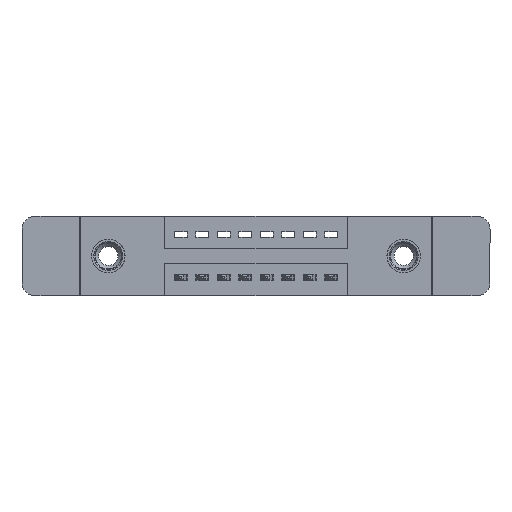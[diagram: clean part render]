
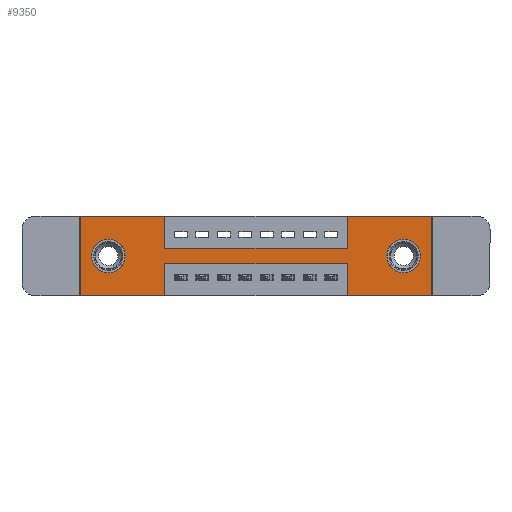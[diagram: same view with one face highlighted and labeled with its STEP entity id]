
A CAD part, front view. The second image highlights one B-rep face of the part: STEP entity #9350.
In plain terms, the highlighted planar face has unit normal (0, -1, 0).
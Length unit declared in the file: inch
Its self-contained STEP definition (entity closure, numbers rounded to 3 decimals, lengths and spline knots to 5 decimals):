
#38 = CARTESIAN_POINT ( 'NONE',  ( 0., 0., 0. ) ) ;
#40 = EDGE_CURVE ( 'NONE', #2316, #5330, #7131, .T. ) ;
#56 = ORIENTED_EDGE ( 'NONE', *, *, #5959, .T. ) ;
#145 = VERTEX_POINT ( 'NONE', #13485 ) ;
#184 = CARTESIAN_POINT ( 'NONE',  ( 0., 0., -0.37 ) ) ;
#198 = EDGE_CURVE ( 'NONE', #11744, #13401, #5810, .T. ) ;
#354 = DIRECTION ( 'NONE',  ( -1., 0., 0. ) ) ;
#569 = CARTESIAN_POINT ( 'NONE',  ( 0.3925, 0., -0.37 ) ) ;
#600 = LINE ( 'NONE', #2339, #7487 ) ;
#678 = VERTEX_POINT ( 'NONE', #4739 ) ;
#805 = EDGE_LOOP ( 'NONE', ( #56, #7225 ) ) ;
#812 = CARTESIAN_POINT ( 'NONE',  ( 0., 0., -0.37 ) ) ;
#832 = LINE ( 'NONE', #38, #14761 ) ;
#871 = AXIS2_PLACEMENT_3D ( 'NONE', #6582, #8857, #4080 ) ;
#1238 = CARTESIAN_POINT ( 'NONE',  ( 1.2425, 0., -0.37 ) ) ;
#1443 = VERTEX_POINT ( 'NONE', #184 ) ;
#1510 = LINE ( 'NONE', #14912, #8026 ) ;
#1944 = CARTESIAN_POINT ( 'NONE',  ( 0.3925, 0., 0. ) ) ;
#2105 = VECTOR ( 'NONE', #10865, 39.37008 ) ;
#2150 = ORIENTED_EDGE ( 'NONE', *, *, #6240, .F. ) ;
#2282 = LINE ( 'NONE', #8129, #6300 ) ;
#2306 = DIRECTION ( 'NONE',  ( 0., 1., 0. ) ) ;
#2316 = VERTEX_POINT ( 'NONE', #6868 ) ;
#2339 = CARTESIAN_POINT ( 'NONE',  ( 0., 0., 0. ) ) ;
#2382 = VECTOR ( 'NONE', #11818, 39.37008 ) ;
#2751 = PLANE ( 'NONE',  #11039 ) ;
#2849 = AXIS2_PLACEMENT_3D ( 'NONE', #15783, #6007, #8430 ) ;
#2877 = EDGE_CURVE ( 'NONE', #6434, #7371, #2282, .T. ) ;
#2977 = VECTOR ( 'NONE', #11588, 39.37008 ) ;
#3133 = VERTEX_POINT ( 'NONE', #12393 ) ;
#3241 = CARTESIAN_POINT ( 'NONE',  ( 0.3925, 0., -0.37 ) ) ;
#3244 = VERTEX_POINT ( 'NONE', #3241 ) ;
#3394 = DIRECTION ( 'NONE',  ( 0., 1., 0. ) ) ;
#3525 = ORIENTED_EDGE ( 'NONE', *, *, #13629, .F. ) ;
#3572 = ORIENTED_EDGE ( 'NONE', *, *, #12669, .T. ) ;
#3719 = VECTOR ( 'NONE', #15218, 39.37008 ) ;
#3744 = ORIENTED_EDGE ( 'NONE', *, *, #6843, .F. ) ;
#4080 = DIRECTION ( 'NONE',  ( 0., 0., -1. ) ) ;
#4309 = ORIENTED_EDGE ( 'NONE', *, *, #15474, .F. ) ;
#4440 = CARTESIAN_POINT ( 'NONE',  ( 0.3925, 0., -0.15 ) ) ;
#4549 = CARTESIAN_POINT ( 'NONE',  ( 0.3925, 0., -0.22 ) ) ;
#4686 = CARTESIAN_POINT ( 'NONE',  ( 0.13, 0., -0.107 ) ) ;
#4704 = DIRECTION ( 'NONE',  ( 0., 0., 1. ) ) ;
#4723 = CIRCLE ( 'NONE', #871, 0.078 ) ;
#4738 = CARTESIAN_POINT ( 'NONE',  ( 0.13, 0., -0.185 ) ) ;
#4739 = CARTESIAN_POINT ( 'NONE',  ( 0., 0., 0. ) ) ;
#5189 = EDGE_LOOP ( 'NONE', ( #3572, #11184 ) ) ;
#5231 = EDGE_LOOP ( 'NONE', ( #10659, #2150, #4309, #3525, #3744, #13785, #8431, #14929, #11423, #13357, #9660, #7241 ) ) ;
#5330 = VERTEX_POINT ( 'NONE', #15211 ) ;
#5810 = CIRCLE ( 'NONE', #9641, 0.078 ) ;
#5941 = LINE ( 'NONE', #569, #10884 ) ;
#5959 = EDGE_CURVE ( 'NONE', #145, #12391, #15179, .T. ) ;
#6007 = DIRECTION ( 'NONE',  ( 0., 1., 0. ) ) ;
#6098 = EDGE_CURVE ( 'NONE', #12391, #145, #4723, .T. ) ;
#6240 = EDGE_CURVE ( 'NONE', #12319, #15354, #14007, .T. ) ;
#6300 = VECTOR ( 'NONE', #13963, 39.37008 ) ;
#6356 = DIRECTION ( 'NONE',  ( 1., 0., 0. ) ) ;
#6434 = VERTEX_POINT ( 'NONE', #10981 ) ;
#6478 = DIRECTION ( 'NONE',  ( 0., -1., 0. ) ) ;
#6488 = VERTEX_POINT ( 'NONE', #15559 ) ;
#6582 = CARTESIAN_POINT ( 'NONE',  ( 1.505, 0., -0.185 ) ) ;
#6825 = FACE_OUTER_BOUND ( 'NONE', #5231, .T. ) ;
#6843 = EDGE_CURVE ( 'NONE', #13503, #3133, #7913, .T. ) ;
#6868 = CARTESIAN_POINT ( 'NONE',  ( 0.3925, 0., 0. ) ) ;
#6890 = DIRECTION ( 'NONE',  ( -1., 0., 0. ) ) ;
#7074 = EDGE_CURVE ( 'NONE', #1443, #678, #14574, .T. ) ;
#7131 = LINE ( 'NONE', #1944, #13185 ) ;
#7144 = CARTESIAN_POINT ( 'NONE',  ( 1.2425, 0., -0.22 ) ) ;
#7225 = ORIENTED_EDGE ( 'NONE', *, *, #6098, .T. ) ;
#7241 = ORIENTED_EDGE ( 'NONE', *, *, #10597, .F. ) ;
#7371 = VERTEX_POINT ( 'NONE', #10656 ) ;
#7487 = VECTOR ( 'NONE', #12174, 39.37008 ) ;
#7728 = VECTOR ( 'NONE', #13560, 39.37008 ) ;
#7837 = DIRECTION ( 'NONE',  ( 0., 0., -1. ) ) ;
#7847 = CARTESIAN_POINT ( 'NONE',  ( 0., 0., 0. ) ) ;
#7913 = LINE ( 'NONE', #12357, #7728 ) ;
#8026 = VECTOR ( 'NONE', #354, 39.37008 ) ;
#8129 = CARTESIAN_POINT ( 'NONE',  ( 1.2425, 0., 0. ) ) ;
#8430 = DIRECTION ( 'NONE',  ( 0., 0., -1. ) ) ;
#8431 = ORIENTED_EDGE ( 'NONE', *, *, #2877, .F. ) ;
#8449 = CARTESIAN_POINT ( 'NONE',  ( 0.13, 0., -0.263 ) ) ;
#8807 = AXIS2_PLACEMENT_3D ( 'NONE', #11964, #3394, #4704 ) ;
#8857 = DIRECTION ( 'NONE',  ( 0., 1., 0. ) ) ;
#8925 = DIRECTION ( 'NONE',  ( 0., 0., -1. ) ) ;
#8977 = LINE ( 'NONE', #1238, #2105 ) ;
#9350 = ADVANCED_FACE ( 'NONE', ( #9682, #10050, #6825 ), #2751, .T. ) ;
#9641 = AXIS2_PLACEMENT_3D ( 'NONE', #4738, #2306, #10839 ) ;
#9660 = ORIENTED_EDGE ( 'NONE', *, *, #7074, .F. ) ;
#9682 = FACE_BOUND ( 'NONE', #805, .T. ) ;
#9731 = DIRECTION ( 'NONE',  ( 0., 0., -1. ) ) ;
#9793 = CARTESIAN_POINT ( 'NONE',  ( 1.505, 0., -0.263 ) ) ;
#10050 = FACE_BOUND ( 'NONE', #5189, .T. ) ;
#10164 = EDGE_CURVE ( 'NONE', #7371, #13503, #832, .T. ) ;
#10530 = EDGE_CURVE ( 'NONE', #5330, #6434, #10585, .T. ) ;
#10585 = LINE ( 'NONE', #4440, #3719 ) ;
#10597 = EDGE_CURVE ( 'NONE', #3244, #1443, #11722, .T. ) ;
#10656 = CARTESIAN_POINT ( 'NONE',  ( 1.2425, 0., 0. ) ) ;
#10659 = ORIENTED_EDGE ( 'NONE', *, *, #13796, .F. ) ;
#10839 = DIRECTION ( 'NONE',  ( 0., 0., 1. ) ) ;
#10865 = DIRECTION ( 'NONE',  ( 0., 0., 1. ) ) ;
#10884 = VECTOR ( 'NONE', #7837, 39.37008 ) ;
#10981 = CARTESIAN_POINT ( 'NONE',  ( 1.2425, 0., -0.15 ) ) ;
#11039 = AXIS2_PLACEMENT_3D ( 'NONE', #12616, #6478, #8925 ) ;
#11184 = ORIENTED_EDGE ( 'NONE', *, *, #198, .T. ) ;
#11423 = ORIENTED_EDGE ( 'NONE', *, *, #40, .F. ) ;
#11588 = DIRECTION ( 'NONE',  ( 0., 0., 1. ) ) ;
#11679 = CIRCLE ( 'NONE', #8807, 0.078 ) ;
#11722 = LINE ( 'NONE', #812, #2382 ) ;
#11744 = VERTEX_POINT ( 'NONE', #8449 ) ;
#11818 = DIRECTION ( 'NONE',  ( -1., 0., 0. ) ) ;
#11964 = CARTESIAN_POINT ( 'NONE',  ( 0.13, 0., -0.185 ) ) ;
#12174 = DIRECTION ( 'NONE',  ( 1., 0., 0. ) ) ;
#12315 = EDGE_CURVE ( 'NONE', #678, #2316, #600, .T. ) ;
#12319 = VERTEX_POINT ( 'NONE', #7144 ) ;
#12357 = CARTESIAN_POINT ( 'NONE',  ( 1.635, 0., 0. ) ) ;
#12391 = VERTEX_POINT ( 'NONE', #9793 ) ;
#12393 = CARTESIAN_POINT ( 'NONE',  ( 1.635, 0., -0.37 ) ) ;
#12616 = CARTESIAN_POINT ( 'NONE',  ( 0., 0., -0.37 ) ) ;
#12669 = EDGE_CURVE ( 'NONE', #13401, #11744, #11679, .T. ) ;
#13185 = VECTOR ( 'NONE', #9731, 39.37008 ) ;
#13357 = ORIENTED_EDGE ( 'NONE', *, *, #12315, .F. ) ;
#13401 = VERTEX_POINT ( 'NONE', #4686 ) ;
#13485 = CARTESIAN_POINT ( 'NONE',  ( 1.505, 0., -0.107 ) ) ;
#13503 = VERTEX_POINT ( 'NONE', #14536 ) ;
#13560 = DIRECTION ( 'NONE',  ( 0., 0., -1. ) ) ;
#13629 = EDGE_CURVE ( 'NONE', #3133, #6488, #1510, .T. ) ;
#13785 = ORIENTED_EDGE ( 'NONE', *, *, #10164, .F. ) ;
#13796 = EDGE_CURVE ( 'NONE', #15354, #3244, #5941, .T. ) ;
#13963 = DIRECTION ( 'NONE',  ( 0., 0., 1. ) ) ;
#14007 = LINE ( 'NONE', #15338, #15544 ) ;
#14536 = CARTESIAN_POINT ( 'NONE',  ( 1.635, 0., 0. ) ) ;
#14574 = LINE ( 'NONE', #7847, #2977 ) ;
#14761 = VECTOR ( 'NONE', #6356, 39.37008 ) ;
#14912 = CARTESIAN_POINT ( 'NONE',  ( 0., 0., -0.37 ) ) ;
#14929 = ORIENTED_EDGE ( 'NONE', *, *, #10530, .F. ) ;
#15179 = CIRCLE ( 'NONE', #2849, 0.078 ) ;
#15211 = CARTESIAN_POINT ( 'NONE',  ( 0.3925, 0., -0.15 ) ) ;
#15218 = DIRECTION ( 'NONE',  ( 1., 0., 0. ) ) ;
#15338 = CARTESIAN_POINT ( 'NONE',  ( 0.3925, 0., -0.22 ) ) ;
#15354 = VERTEX_POINT ( 'NONE', #4549 ) ;
#15474 = EDGE_CURVE ( 'NONE', #6488, #12319, #8977, .T. ) ;
#15544 = VECTOR ( 'NONE', #6890, 39.37008 ) ;
#15559 = CARTESIAN_POINT ( 'NONE',  ( 1.2425, 0., -0.37 ) ) ;
#15783 = CARTESIAN_POINT ( 'NONE',  ( 1.505, 0., -0.185 ) ) ;
